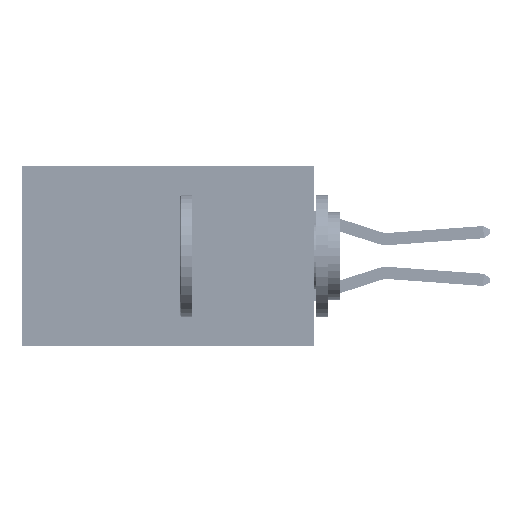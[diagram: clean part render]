
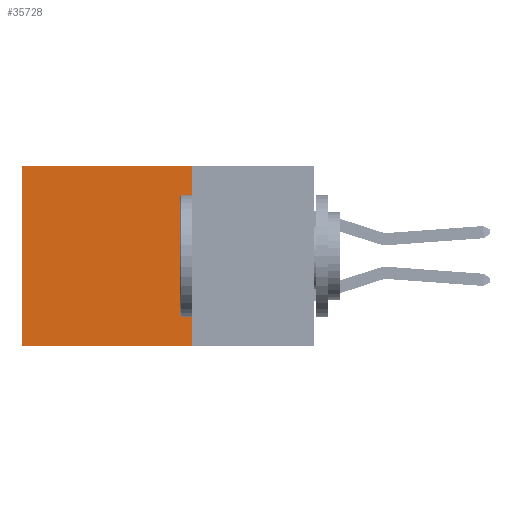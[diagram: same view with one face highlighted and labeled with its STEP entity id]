
A CAD part, left-side view. The second image highlights one B-rep face of the part: STEP entity #35728.
In plain terms, the highlighted planar face has unit normal (-1, 0, 0).
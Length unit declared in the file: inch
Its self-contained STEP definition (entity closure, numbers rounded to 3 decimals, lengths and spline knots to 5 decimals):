
#2123 = VERTEX_POINT ( 'NONE', #38444 ) ;
#2145 = EDGE_CURVE ( 'NONE', #50273, #18460, #21089, .T. ) ;
#3573 = CARTESIAN_POINT ( 'NONE',  ( 0.2875, 0.25, 0. ) ) ;
#5612 = ORIENTED_EDGE ( 'NONE', *, *, #2145, .T. ) ;
#6364 = CARTESIAN_POINT ( 'NONE',  ( 0.2875, 0.6, -0.37 ) ) ;
#7439 = ORIENTED_EDGE ( 'NONE', *, *, #13794, .T. ) ;
#7637 = AXIS2_PLACEMENT_3D ( 'NONE', #3573, #44581, #20261 ) ;
#10704 = DIRECTION ( 'NONE',  ( 0., 0., -1. ) ) ;
#11313 = LINE ( 'NONE', #32181, #31057 ) ;
#11947 = DIRECTION ( 'NONE',  ( 0., 0., -1. ) ) ;
#13794 = EDGE_CURVE ( 'NONE', #32118, #50273, #11313, .T. ) ;
#14534 = DIRECTION ( 'NONE',  ( 0., 1., 0. ) ) ;
#16172 = PLANE ( 'NONE',  #7637 ) ;
#17108 = CARTESIAN_POINT ( 'NONE',  ( 0.2875, 0.6, 0. ) ) ;
#18402 = EDGE_CURVE ( 'NONE', #2123, #18460, #37805, .T. ) ;
#18460 = VERTEX_POINT ( 'NONE', #6364 ) ;
#20261 = DIRECTION ( 'NONE',  ( 0., 0., -1. ) ) ;
#20305 = DIRECTION ( 'NONE',  ( 0., 1., 0. ) ) ;
#21089 = LINE ( 'NONE', #50843, #36974 ) ;
#24212 = FACE_OUTER_BOUND ( 'NONE', #45924, .T. ) ;
#26174 = ORIENTED_EDGE ( 'NONE', *, *, #33692, .F. ) ;
#26277 = CARTESIAN_POINT ( 'NONE',  ( 0.2875, 0.25, -0.37 ) ) ;
#29642 = VECTOR ( 'NONE', #11947, 39.37008 ) ;
#29954 = ORIENTED_EDGE ( 'NONE', *, *, #18402, .F. ) ;
#31057 = VECTOR ( 'NONE', #20305, 39.37008 ) ;
#31517 = LINE ( 'NONE', #44270, #29642 ) ;
#32118 = VERTEX_POINT ( 'NONE', #41338 ) ;
#32181 = CARTESIAN_POINT ( 'NONE',  ( 0.2875, 0.25, 0. ) ) ;
#33372 = VECTOR ( 'NONE', #14534, 39.37008 ) ;
#33692 = EDGE_CURVE ( 'NONE', #32118, #2123, #31517, .T. ) ;
#35728 = ADVANCED_FACE ( 'NONE', ( #24212 ), #16172, .F. ) ;
#36974 = VECTOR ( 'NONE', #10704, 39.37008 ) ;
#37805 = LINE ( 'NONE', #26277, #33372 ) ;
#38444 = CARTESIAN_POINT ( 'NONE',  ( 0.2875, 0.25, -0.37 ) ) ;
#41338 = CARTESIAN_POINT ( 'NONE',  ( 0.2875, 0.25, 0. ) ) ;
#44270 = CARTESIAN_POINT ( 'NONE',  ( 0.2875, 0.25, 0. ) ) ;
#44581 = DIRECTION ( 'NONE',  ( 1., 0., 0. ) ) ;
#45924 = EDGE_LOOP ( 'NONE', ( #5612, #29954, #26174, #7439 ) ) ;
#50273 = VERTEX_POINT ( 'NONE', #17108 ) ;
#50843 = CARTESIAN_POINT ( 'NONE',  ( 0.2875, 0.6, 0. ) ) ;
